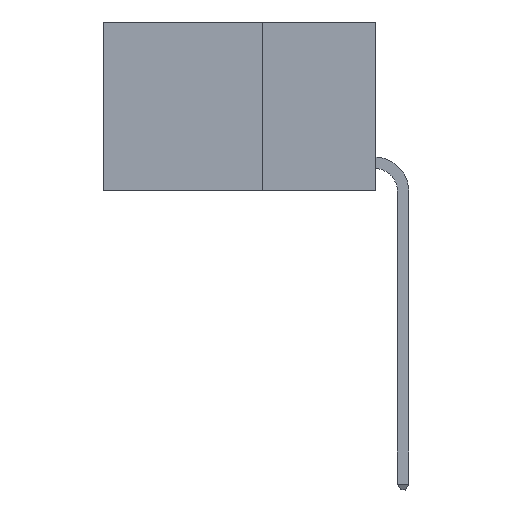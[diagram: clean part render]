
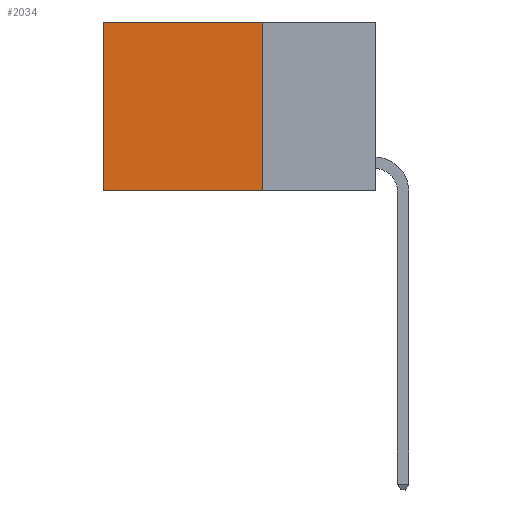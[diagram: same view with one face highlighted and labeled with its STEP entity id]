
A CAD part, left-side view. The second image highlights one B-rep face of the part: STEP entity #2034.
In plain terms, the highlighted planar face has unit normal (-1, 0, 0).
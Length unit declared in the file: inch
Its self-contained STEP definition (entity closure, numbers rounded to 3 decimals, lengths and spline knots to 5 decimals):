
#428 = DIRECTION ( 'NONE',  ( 0., 0., -1. ) ) ;
#619 = EDGE_LOOP ( 'NONE', ( #3656, #3726, #4472, #4795 ) ) ;
#1021 = LINE ( 'NONE', #8623, #5670 ) ;
#2034 = ADVANCED_FACE ( 'NONE', ( #7235 ), #7835, .F. ) ;
#2575 = DIRECTION ( 'NONE',  ( 0., 1., 0. ) ) ;
#2653 = DIRECTION ( 'NONE',  ( 0., 0., -1. ) ) ;
#2877 = VERTEX_POINT ( 'NONE', #7050 ) ;
#3319 = VECTOR ( 'NONE', #3588, 39.37008 ) ;
#3588 = DIRECTION ( 'NONE',  ( 0., 1., 0. ) ) ;
#3656 = ORIENTED_EDGE ( 'NONE', *, *, #9476, .T. ) ;
#3726 = ORIENTED_EDGE ( 'NONE', *, *, #4827, .F. ) ;
#3728 = LINE ( 'NONE', #9324, #7678 ) ;
#3886 = CARTESIAN_POINT ( 'NONE',  ( 0.2625, 0.6, 0. ) ) ;
#4170 = VERTEX_POINT ( 'NONE', #11000 ) ;
#4472 = ORIENTED_EDGE ( 'NONE', *, *, #7861, .F. ) ;
#4620 = VECTOR ( 'NONE', #428, 39.37008 ) ;
#4627 = AXIS2_PLACEMENT_3D ( 'NONE', #4719, #9422, #9391 ) ;
#4719 = CARTESIAN_POINT ( 'NONE',  ( 0.2625, 0.25, 0. ) ) ;
#4795 = ORIENTED_EDGE ( 'NONE', *, *, #9445, .T. ) ;
#4827 = EDGE_CURVE ( 'NONE', #2877, #4170, #3728, .T. ) ;
#5103 = VERTEX_POINT ( 'NONE', #3886 ) ;
#5182 = CARTESIAN_POINT ( 'NONE',  ( 0.2625, 0.25, 0. ) ) ;
#5670 = VECTOR ( 'NONE', #2653, 39.37008 ) ;
#5907 = VERTEX_POINT ( 'NONE', #5182 ) ;
#5929 = LINE ( 'NONE', #7784, #3319 ) ;
#7050 = CARTESIAN_POINT ( 'NONE',  ( 0.2625, 0.25, -0.37 ) ) ;
#7235 = FACE_OUTER_BOUND ( 'NONE', #619, .T. ) ;
#7678 = VECTOR ( 'NONE', #2575, 39.37008 ) ;
#7784 = CARTESIAN_POINT ( 'NONE',  ( 0.2625, 0.25, 0. ) ) ;
#7835 = PLANE ( 'NONE',  #4627 ) ;
#7861 = EDGE_CURVE ( 'NONE', #5907, #2877, #8736, .T. ) ;
#8623 = CARTESIAN_POINT ( 'NONE',  ( 0.2625, 0.6, 0. ) ) ;
#8736 = LINE ( 'NONE', #10740, #4620 ) ;
#9324 = CARTESIAN_POINT ( 'NONE',  ( 0.2625, 0.25, -0.37 ) ) ;
#9391 = DIRECTION ( 'NONE',  ( 0., 0., -1. ) ) ;
#9422 = DIRECTION ( 'NONE',  ( 1., 0., 0. ) ) ;
#9445 = EDGE_CURVE ( 'NONE', #5907, #5103, #5929, .T. ) ;
#9476 = EDGE_CURVE ( 'NONE', #5103, #4170, #1021, .T. ) ;
#10740 = CARTESIAN_POINT ( 'NONE',  ( 0.2625, 0.25, 0. ) ) ;
#11000 = CARTESIAN_POINT ( 'NONE',  ( 0.2625, 0.6, -0.37 ) ) ;
